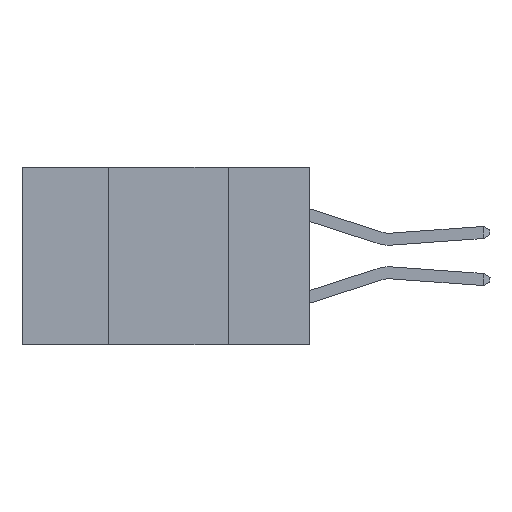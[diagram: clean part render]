
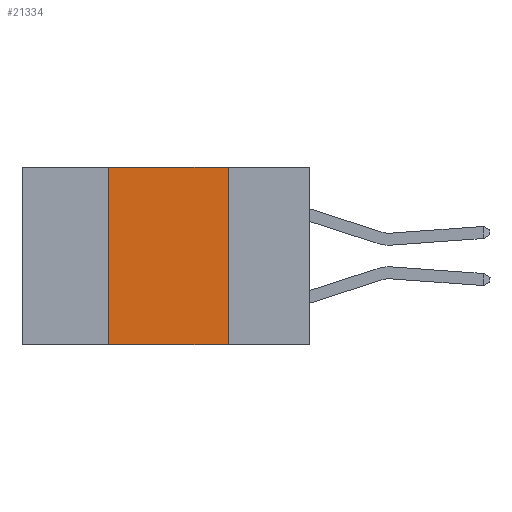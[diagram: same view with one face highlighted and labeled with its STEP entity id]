
A CAD part, left-side view. The second image highlights one B-rep face of the part: STEP entity #21334.
In plain terms, the highlighted planar face has unit normal (-1, 0, 0).
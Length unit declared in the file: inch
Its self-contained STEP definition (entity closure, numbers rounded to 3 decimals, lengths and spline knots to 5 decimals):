
#1206 = EDGE_CURVE ( 'NONE', #5108, #15970, #19959, .T. ) ;
#1260 = ORIENTED_EDGE ( 'NONE', *, *, #1206, .F. ) ;
#1660 = CARTESIAN_POINT ( 'NONE',  ( 0., 0.42, -0.37 ) ) ;
#3538 = CARTESIAN_POINT ( 'NONE',  ( 0., 0.6, -0.37 ) ) ;
#3682 = VECTOR ( 'NONE', #10929, 39.37008 ) ;
#3945 = VECTOR ( 'NONE', #23550, 39.37008 ) ;
#5108 = VERTEX_POINT ( 'NONE', #1660 ) ;
#7488 = EDGE_CURVE ( 'NONE', #25875, #17415, #10801, .T. ) ;
#9342 = CARTESIAN_POINT ( 'NONE',  ( 0., 0.6, 0. ) ) ;
#9423 = EDGE_CURVE ( 'NONE', #15970, #25875, #15471, .T. ) ;
#10062 = CARTESIAN_POINT ( 'NONE',  ( 0., 0.17, -0.37 ) ) ;
#10732 = DIRECTION ( 'NONE',  ( 1., 0., 0. ) ) ;
#10801 = LINE ( 'NONE', #10062, #26284 ) ;
#10895 = ORIENTED_EDGE ( 'NONE', *, *, #9423, .F. ) ;
#10929 = DIRECTION ( 'NONE',  ( 0., 0., 1. ) ) ;
#10975 = CARTESIAN_POINT ( 'NONE',  ( 0., 0.42, -0.37 ) ) ;
#12252 = EDGE_CURVE ( 'NONE', #5108, #17415, #18810, .T. ) ;
#12811 = ORIENTED_EDGE ( 'NONE', *, *, #12252, .T. ) ;
#12971 = EDGE_LOOP ( 'NONE', ( #25151, #10895, #1260, #12811 ) ) ;
#14743 = PLANE ( 'NONE',  #22695 ) ;
#15471 = LINE ( 'NONE', #9342, #3945 ) ;
#15859 = DIRECTION ( 'NONE',  ( 0., -1., 0. ) ) ;
#15970 = VERTEX_POINT ( 'NONE', #19167 ) ;
#16203 = DIRECTION ( 'NONE',  ( 0., 0., -1. ) ) ;
#17415 = VERTEX_POINT ( 'NONE', #21651 ) ;
#18810 = LINE ( 'NONE', #3538, #25029 ) ;
#19167 = CARTESIAN_POINT ( 'NONE',  ( 0., 0.42, 0. ) ) ;
#19959 = LINE ( 'NONE', #10975, #3682 ) ;
#20821 = FACE_OUTER_BOUND ( 'NONE', #12971, .T. ) ;
#20869 = CARTESIAN_POINT ( 'NONE',  ( 0., 0.6, 0. ) ) ;
#21334 = ADVANCED_FACE ( 'NONE', ( #20821 ), #14743, .F. ) ;
#21651 = CARTESIAN_POINT ( 'NONE',  ( 0., 0.17, -0.37 ) ) ;
#22695 = AXIS2_PLACEMENT_3D ( 'NONE', #20869, #10732, #24874 ) ;
#23550 = DIRECTION ( 'NONE',  ( 0., -1., 0. ) ) ;
#24585 = CARTESIAN_POINT ( 'NONE',  ( 0., 0.17, 0. ) ) ;
#24874 = DIRECTION ( 'NONE',  ( 0., 0., -1. ) ) ;
#25029 = VECTOR ( 'NONE', #15859, 39.37008 ) ;
#25151 = ORIENTED_EDGE ( 'NONE', *, *, #7488, .F. ) ;
#25875 = VERTEX_POINT ( 'NONE', #24585 ) ;
#26284 = VECTOR ( 'NONE', #16203, 39.37008 ) ;
